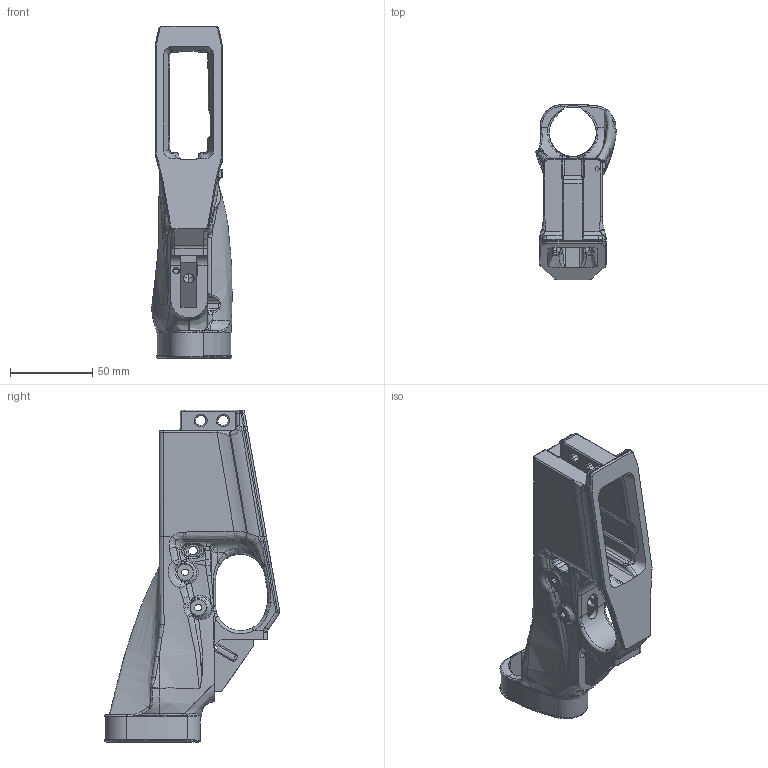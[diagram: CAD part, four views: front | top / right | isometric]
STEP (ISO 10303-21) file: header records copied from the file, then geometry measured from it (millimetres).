
FILE_DESCRIPTION (( 'STEP AP203' ), '1' );
FILE_NAME ('Super AR-15 Lower V3.0.STEP', '2021-11-11T22:56:28', ( '' ), ( '' ), 'SwSTEP 2.0', 'SolidWorks 2021', '' );
FILE_SCHEMA (( 'CONFIG_CONTROL_DESIGN' ));
Products named in the file (1): Super AR-15 Lower V3.0
Bounding box: 48.78 x 106.75 x 201.55 mm (x, y, z)
Volume: 177824.2 mm3; surface area: 65282.8 mm2
Topology: 1 solids, 1 shells, 1799 faces, 4725 edges, 2947 vertices
Faces by surface type: bspline 749, plane 555, cylinder 341, torus 106, cone 32, sphere 16
Entity records: 112673 total; most frequent: CARTESIAN_POINT 74428, ORIENTED_EDGE 9368, DIRECTION 5878, EDGE_CURVE 4684, VERTEX_POINT 2947, AXIS2_PLACEMENT_3D 1989, EDGE_LOOP 1901, LINE 1900
